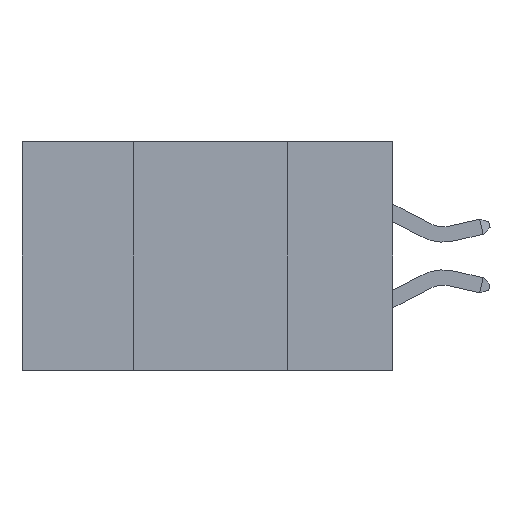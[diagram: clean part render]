
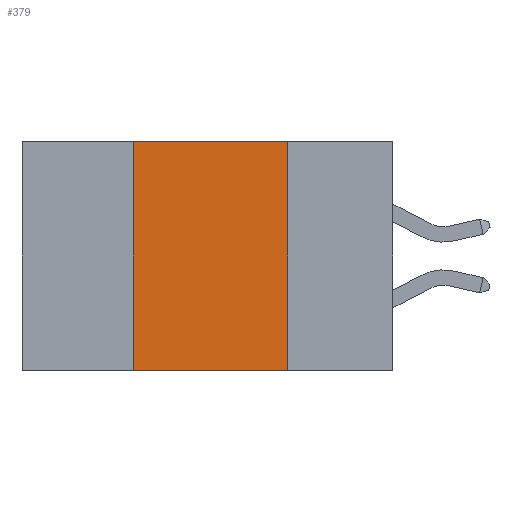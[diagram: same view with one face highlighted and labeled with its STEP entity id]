
A CAD part, left-side view. The second image highlights one B-rep face of the part: STEP entity #379.
In plain terms, the highlighted planar face has unit normal (-1, 0, 0).
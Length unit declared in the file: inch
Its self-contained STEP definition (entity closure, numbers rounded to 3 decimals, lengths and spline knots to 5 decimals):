
#271 = DIRECTION ( 'NONE',  ( 0., -1., 0. ) ) ;
#379 = ADVANCED_FACE ( 'NONE', ( #14181 ), #13852, .F. ) ;
#407 = DIRECTION ( 'NONE',  ( 1., 0., 0. ) ) ;
#751 = VECTOR ( 'NONE', #4144, 39.37008 ) ;
#1437 = DIRECTION ( 'NONE',  ( 0., 0., -1. ) ) ;
#2088 = ORIENTED_EDGE ( 'NONE', *, *, #12882, .F. ) ;
#2262 = CARTESIAN_POINT ( 'NONE',  ( 0., 0.42, 0. ) ) ;
#2917 = EDGE_CURVE ( 'NONE', #12600, #12781, #11694, .T. ) ;
#3659 = LINE ( 'NONE', #2262, #5425 ) ;
#4006 = CARTESIAN_POINT ( 'NONE',  ( 0., 0.6, 0. ) ) ;
#4144 = DIRECTION ( 'NONE',  ( 0., -1., 0. ) ) ;
#5036 = CARTESIAN_POINT ( 'NONE',  ( 0., 0.17, 0. ) ) ;
#5122 = CARTESIAN_POINT ( 'NONE',  ( 0., 0.6, -0.37 ) ) ;
#5425 = VECTOR ( 'NONE', #13743, 39.37008 ) ;
#6874 = ORIENTED_EDGE ( 'NONE', *, *, #15770, .F. ) ;
#6914 = CARTESIAN_POINT ( 'NONE',  ( 0., 0.17, 0. ) ) ;
#7144 = ORIENTED_EDGE ( 'NONE', *, *, #7285, .F. ) ;
#7285 = EDGE_CURVE ( 'NONE', #8827, #12781, #15286, .T. ) ;
#7975 = LINE ( 'NONE', #9043, #15647 ) ;
#8827 = VERTEX_POINT ( 'NONE', #6914 ) ;
#9043 = CARTESIAN_POINT ( 'NONE',  ( 0., 0.6, 0. ) ) ;
#9647 = AXIS2_PLACEMENT_3D ( 'NONE', #4006, #407, #12792 ) ;
#10268 = VERTEX_POINT ( 'NONE', #11173 ) ;
#11173 = CARTESIAN_POINT ( 'NONE',  ( 0., 0.42, 0. ) ) ;
#11694 = LINE ( 'NONE', #5122, #751 ) ;
#11863 = EDGE_LOOP ( 'NONE', ( #7144, #2088, #6874, #13779 ) ) ;
#12600 = VERTEX_POINT ( 'NONE', #13075 ) ;
#12781 = VERTEX_POINT ( 'NONE', #13714 ) ;
#12792 = DIRECTION ( 'NONE',  ( 0., 0., -1. ) ) ;
#12882 = EDGE_CURVE ( 'NONE', #10268, #8827, #7975, .T. ) ;
#13075 = CARTESIAN_POINT ( 'NONE',  ( 0., 0.42, -0.37 ) ) ;
#13714 = CARTESIAN_POINT ( 'NONE',  ( 0., 0.17, -0.37 ) ) ;
#13743 = DIRECTION ( 'NONE',  ( 0., 0., 1. ) ) ;
#13779 = ORIENTED_EDGE ( 'NONE', *, *, #2917, .T. ) ;
#13852 = PLANE ( 'NONE',  #9647 ) ;
#14181 = FACE_OUTER_BOUND ( 'NONE', #11863, .T. ) ;
#14182 = VECTOR ( 'NONE', #1437, 39.37008 ) ;
#15286 = LINE ( 'NONE', #5036, #14182 ) ;
#15647 = VECTOR ( 'NONE', #271, 39.37008 ) ;
#15770 = EDGE_CURVE ( 'NONE', #12600, #10268, #3659, .T. ) ;
